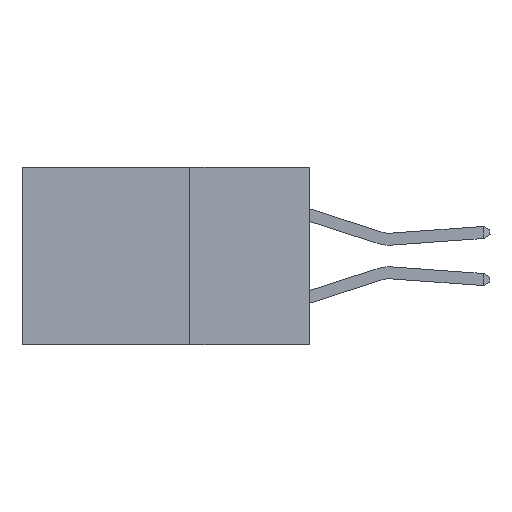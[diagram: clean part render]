
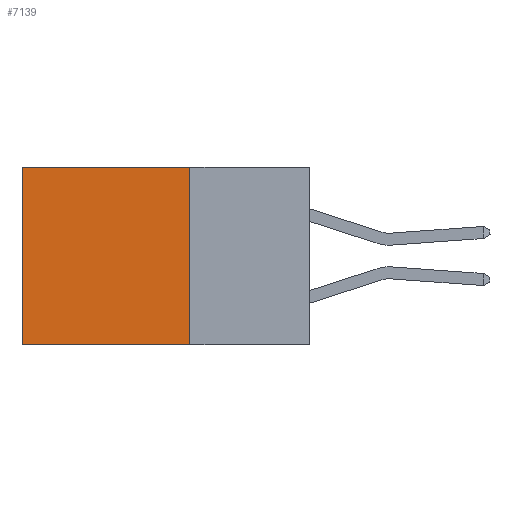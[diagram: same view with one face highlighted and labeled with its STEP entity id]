
A CAD part, left-side view. The second image highlights one B-rep face of the part: STEP entity #7139.
In plain terms, the highlighted planar face has unit normal (-1, 0, 0).
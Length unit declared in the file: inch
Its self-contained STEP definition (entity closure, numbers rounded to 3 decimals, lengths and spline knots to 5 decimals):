
#1214 = CARTESIAN_POINT ( 'NONE',  ( 0.298, 0.6, 0. ) ) ;
#2299 = VECTOR ( 'NONE', #5949, 39.37008 ) ;
#2313 = EDGE_LOOP ( 'NONE', ( #9718, #3204, #13815, #8560 ) ) ;
#2451 = VECTOR ( 'NONE', #6016, 39.37008 ) ;
#2463 = VECTOR ( 'NONE', #6516, 39.37008 ) ;
#2790 = DIRECTION ( 'NONE',  ( 0., 0., -1. ) ) ;
#3074 = AXIS2_PLACEMENT_3D ( 'NONE', #9045, #5972, #17031 ) ;
#3204 = ORIENTED_EDGE ( 'NONE', *, *, #9385, .F. ) ;
#4955 = CARTESIAN_POINT ( 'NONE',  ( 0.298, 0.25, -0.37 ) ) ;
#5949 = DIRECTION ( 'NONE',  ( 0., 0., -1. ) ) ;
#5972 = DIRECTION ( 'NONE',  ( 1., 0., 0. ) ) ;
#6016 = DIRECTION ( 'NONE',  ( 0., 1., 0. ) ) ;
#6394 = LINE ( 'NONE', #18472, #2299 ) ;
#6516 = DIRECTION ( 'NONE',  ( 0., 1., 0. ) ) ;
#6942 = CARTESIAN_POINT ( 'NONE',  ( 0.298, 0.6, -0.37 ) ) ;
#7116 = VECTOR ( 'NONE', #2790, 39.37008 ) ;
#7139 = ADVANCED_FACE ( 'NONE', ( #14638 ), #16959, .F. ) ;
#7554 = LINE ( 'NONE', #4955, #2463 ) ;
#7660 = VERTEX_POINT ( 'NONE', #18077 ) ;
#7831 = EDGE_CURVE ( 'NONE', #17776, #11992, #6394, .T. ) ;
#8560 = ORIENTED_EDGE ( 'NONE', *, *, #16297, .T. ) ;
#9045 = CARTESIAN_POINT ( 'NONE',  ( 0.298, 0.25, 0. ) ) ;
#9385 = EDGE_CURVE ( 'NONE', #11992, #19822, #7554, .T. ) ;
#9718 = ORIENTED_EDGE ( 'NONE', *, *, #14527, .T. ) ;
#11992 = VERTEX_POINT ( 'NONE', #15629 ) ;
#13815 = ORIENTED_EDGE ( 'NONE', *, *, #7831, .F. ) ;
#13948 = CARTESIAN_POINT ( 'NONE',  ( 0.298, 0.25, 0. ) ) ;
#14527 = EDGE_CURVE ( 'NONE', #7660, #19822, #20156, .T. ) ;
#14638 = FACE_OUTER_BOUND ( 'NONE', #2313, .T. ) ;
#15629 = CARTESIAN_POINT ( 'NONE',  ( 0.298, 0.25, -0.37 ) ) ;
#16297 = EDGE_CURVE ( 'NONE', #17776, #7660, #19137, .T. ) ;
#16959 = PLANE ( 'NONE',  #3074 ) ;
#17031 = DIRECTION ( 'NONE',  ( 0., 0., -1. ) ) ;
#17502 = CARTESIAN_POINT ( 'NONE',  ( 0.298, 0.25, 0. ) ) ;
#17776 = VERTEX_POINT ( 'NONE', #17502 ) ;
#18077 = CARTESIAN_POINT ( 'NONE',  ( 0.298, 0.6, 0. ) ) ;
#18472 = CARTESIAN_POINT ( 'NONE',  ( 0.298, 0.25, 0. ) ) ;
#19137 = LINE ( 'NONE', #13948, #2451 ) ;
#19822 = VERTEX_POINT ( 'NONE', #6942 ) ;
#20156 = LINE ( 'NONE', #1214, #7116 ) ;
